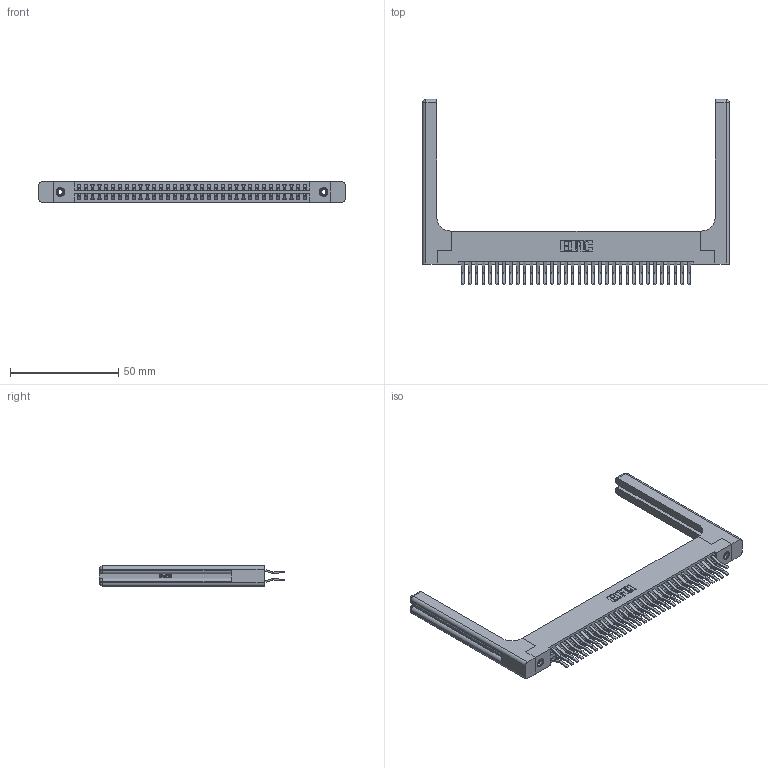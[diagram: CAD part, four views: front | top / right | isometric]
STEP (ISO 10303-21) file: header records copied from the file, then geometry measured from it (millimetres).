
FILE_DESCRIPTION (( 'STEP AP203' ), '1' );
FILE_NAME ('346-068-560-258.STEP', '2022-05-24T20:25:08', ( '' ), ( '' ), 'SwSTEP 2.0', 'SolidWorks 2020', '' );
FILE_SCHEMA (( 'CONFIG_CONTROL_DESIGN' ));
Length unit declared in the file: inch
Products named in the file (5): 345-250-001_345-250-001-102; 346 Part_Flush Mounting Lugs - 0.156 Dia-TH; 345-292-001_560 Tail; 346-068-560-258; 346-220-058_345-220-058
Assembly tree (73 placements, depth 2):
  346-068-560-258
    346 Part_Flush Mounting Lugs - 0.156 Dia-TH
    345-292-001_560 Tail  x68
    345-250-001_345-250-001-102  x2
    346-220-058_345-220-058  x2
Bounding box: 142.01 x 85.74 x 9.4 mm (x, y, z)
Volume: 21707.6 mm3; surface area: 25607.9 mm2
Topology: 73 solids, 73 shells, 4064 faces, 11979 edges, 7874 vertices
Faces by surface type: plane 2618, cylinder 1386, bspline 36, cone 12, sphere 8, torus 4
Entity records: 28952 total; most frequent: CARTESIAN_POINT 5795, ORIENTED_EDGE 4524, DIRECTION 4094, EDGE_CURVE 2262, LINE 1898, VECTOR 1898, VERTEX_POINT 1498, AXIS2_PLACEMENT_3D 1098
